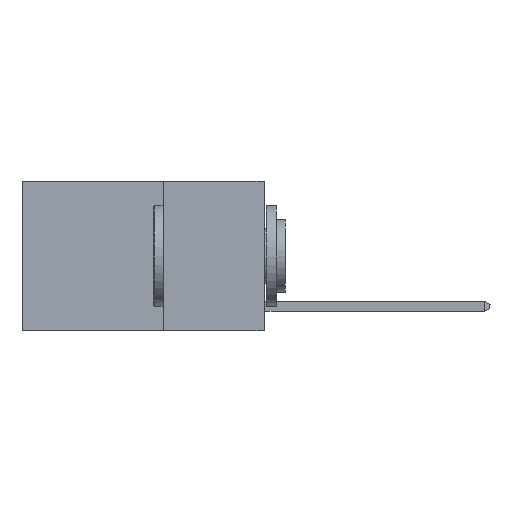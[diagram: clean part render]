
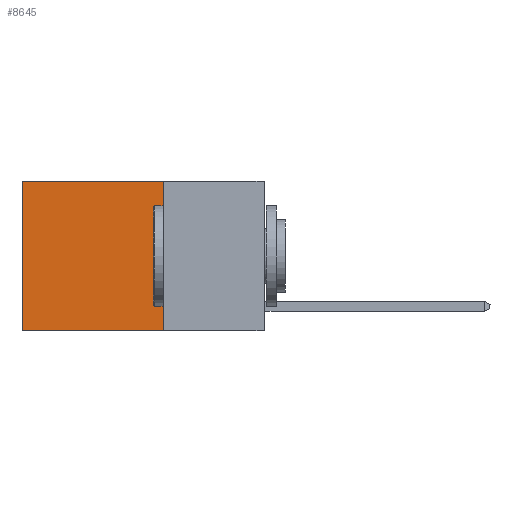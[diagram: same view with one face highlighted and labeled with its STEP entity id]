
A CAD part, left-side view. The second image highlights one B-rep face of the part: STEP entity #8645.
In plain terms, the highlighted planar face has unit normal (-1, 0, 0).
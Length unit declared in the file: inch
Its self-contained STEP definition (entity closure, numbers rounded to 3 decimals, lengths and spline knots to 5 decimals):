
#28 = VECTOR ( 'NONE', #950, 39.37008 ) ;
#135 = VERTEX_POINT ( 'NONE', #5025 ) ;
#223 = FACE_OUTER_BOUND ( 'NONE', #1897, .T. ) ;
#795 = EDGE_CURVE ( 'NONE', #11090, #135, #8335, .T. ) ;
#950 = DIRECTION ( 'NONE',  ( 0., 1., 0. ) ) ;
#1141 = DIRECTION ( 'NONE',  ( 1., 0., 0. ) ) ;
#1502 = VECTOR ( 'NONE', #4795, 39.37008 ) ;
#1757 = AXIS2_PLACEMENT_3D ( 'NONE', #1955, #1141, #7434 ) ;
#1897 = EDGE_LOOP ( 'NONE', ( #10023, #6151, #9451, #2254 ) ) ;
#1955 = CARTESIAN_POINT ( 'NONE',  ( 0.2625, 0.25, 0. ) ) ;
#2254 = ORIENTED_EDGE ( 'NONE', *, *, #2276, .T. ) ;
#2276 = EDGE_CURVE ( 'NONE', #5659, #9732, #10247, .T. ) ;
#2892 = VECTOR ( 'NONE', #5087, 39.37008 ) ;
#2906 = CARTESIAN_POINT ( 'NONE',  ( 0.2625, 0.25, 0. ) ) ;
#4539 = CARTESIAN_POINT ( 'NONE',  ( 0.2625, 0.25, 0. ) ) ;
#4795 = DIRECTION ( 'NONE',  ( 0., 1., 0. ) ) ;
#4967 = CARTESIAN_POINT ( 'NONE',  ( 0.2625, 0.25, -0.37 ) ) ;
#5022 = LINE ( 'NONE', #6037, #2892 ) ;
#5025 = CARTESIAN_POINT ( 'NONE',  ( 0.2625, 0.6, -0.37 ) ) ;
#5087 = DIRECTION ( 'NONE',  ( 0., 0., -1. ) ) ;
#5659 = VERTEX_POINT ( 'NONE', #11484 ) ;
#5849 = VECTOR ( 'NONE', #8052, 39.37008 ) ;
#6037 = CARTESIAN_POINT ( 'NONE',  ( 0.2625, 0.6, 0. ) ) ;
#6151 = ORIENTED_EDGE ( 'NONE', *, *, #795, .F. ) ;
#6586 = PLANE ( 'NONE',  #1757 ) ;
#7434 = DIRECTION ( 'NONE',  ( 0., 0., -1. ) ) ;
#7937 = EDGE_CURVE ( 'NONE', #5659, #11090, #9548, .T. ) ;
#8052 = DIRECTION ( 'NONE',  ( 0., 0., -1. ) ) ;
#8056 = EDGE_CURVE ( 'NONE', #9732, #135, #5022, .T. ) ;
#8335 = LINE ( 'NONE', #10958, #28 ) ;
#8645 = ADVANCED_FACE ( 'NONE', ( #223 ), #6586, .F. ) ;
#9451 = ORIENTED_EDGE ( 'NONE', *, *, #7937, .F. ) ;
#9548 = LINE ( 'NONE', #4539, #5849 ) ;
#9732 = VERTEX_POINT ( 'NONE', #11538 ) ;
#10023 = ORIENTED_EDGE ( 'NONE', *, *, #8056, .T. ) ;
#10247 = LINE ( 'NONE', #2906, #1502 ) ;
#10958 = CARTESIAN_POINT ( 'NONE',  ( 0.2625, 0.25, -0.37 ) ) ;
#11090 = VERTEX_POINT ( 'NONE', #4967 ) ;
#11484 = CARTESIAN_POINT ( 'NONE',  ( 0.2625, 0.25, 0. ) ) ;
#11538 = CARTESIAN_POINT ( 'NONE',  ( 0.2625, 0.6, 0. ) ) ;
